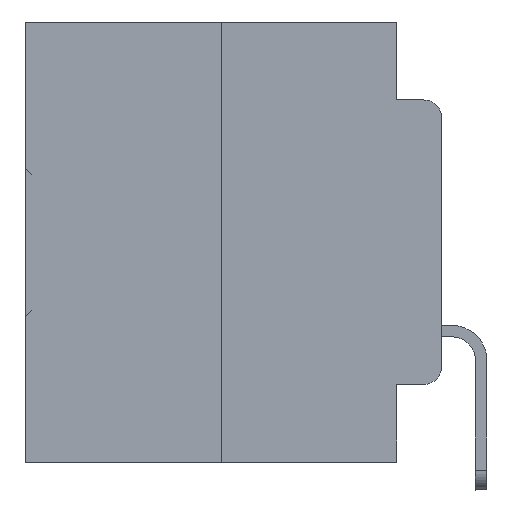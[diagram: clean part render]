
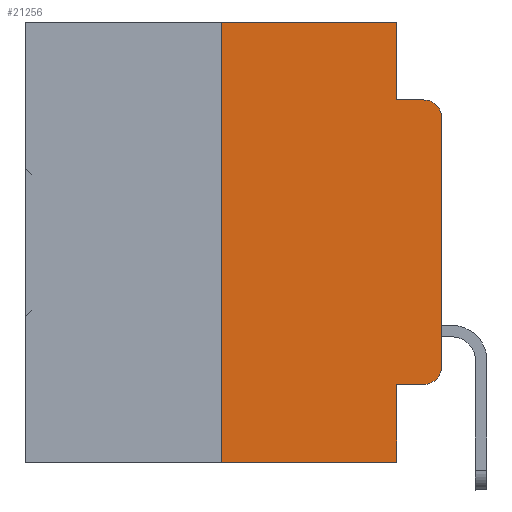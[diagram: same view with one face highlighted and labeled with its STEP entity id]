
A CAD part, left-side view. The second image highlights one B-rep face of the part: STEP entity #21256.
In plain terms, the highlighted planar face has unit normal (-1, 0, 0).
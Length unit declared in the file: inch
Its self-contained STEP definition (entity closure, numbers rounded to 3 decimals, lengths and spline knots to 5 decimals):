
#494 = CARTESIAN_POINT ( 'NONE',  ( 0., 0.02, -0.4115 ) ) ;
#692 = LINE ( 'NONE', #28196, #25234 ) ;
#1241 = CARTESIAN_POINT ( 'NONE',  ( 0., 0.25, 0. ) ) ;
#1628 = VECTOR ( 'NONE', #8132, 39.37008 ) ;
#1717 = EDGE_CURVE ( 'NONE', #23612, #13512, #17549, .T. ) ;
#2669 = EDGE_CURVE ( 'NONE', #31862, #13512, #12969, .T. ) ;
#2868 = ORIENTED_EDGE ( 'NONE', *, *, #9686, .F. ) ;
#3126 = AXIS2_PLACEMENT_3D ( 'NONE', #11331, #33373, #30530 ) ;
#3228 = FACE_OUTER_BOUND ( 'NONE', #25958, .T. ) ;
#3734 = ORIENTED_EDGE ( 'NONE', *, *, #23345, .F. ) ;
#3857 = DIRECTION ( 'NONE',  ( 0., -1., 0. ) ) ;
#3960 = VERTEX_POINT ( 'NONE', #15705 ) ;
#4089 = CIRCLE ( 'NONE', #10333, 0.02 ) ;
#4137 = DIRECTION ( 'NONE',  ( 0., 0., -1. ) ) ;
#4285 = ORIENTED_EDGE ( 'NONE', *, *, #2669, .F. ) ;
#4407 = VERTEX_POINT ( 'NONE', #11495 ) ;
#6607 = CARTESIAN_POINT ( 'NONE',  ( 0., 0.473, 0. ) ) ;
#7118 = LINE ( 'NONE', #12787, #20910 ) ;
#7383 = EDGE_CURVE ( 'NONE', #31862, #33399, #21274, .T. ) ;
#7499 = ORIENTED_EDGE ( 'NONE', *, *, #1717, .T. ) ;
#8031 = VECTOR ( 'NONE', #4137, 39.37008 ) ;
#8132 = DIRECTION ( 'NONE',  ( 0., -1., 0. ) ) ;
#8559 = PLANE ( 'NONE',  #22183 ) ;
#8773 = ORIENTED_EDGE ( 'NONE', *, *, #21470, .T. ) ;
#9200 = CARTESIAN_POINT ( 'NONE',  ( 0., 0.051, -0.4115 ) ) ;
#9288 = VECTOR ( 'NONE', #19876, 39.37008 ) ;
#9291 = CARTESIAN_POINT ( 'NONE',  ( 0., 0., 0. ) ) ;
#9639 = LINE ( 'NONE', #28285, #8031 ) ;
#9686 = EDGE_CURVE ( 'NONE', #28482, #16308, #9639, .T. ) ;
#9745 = EDGE_CURVE ( 'NONE', #4407, #3960, #33645, .T. ) ;
#9904 = CARTESIAN_POINT ( 'NONE',  ( 0., 0.473, -0.5 ) ) ;
#10333 = AXIS2_PLACEMENT_3D ( 'NONE', #20625, #31488, #17977 ) ;
#11331 = CARTESIAN_POINT ( 'NONE',  ( 0., 0.02, -0.3915 ) ) ;
#11495 = CARTESIAN_POINT ( 'NONE',  ( 0., 0., -0.3915 ) ) ;
#11615 = ORIENTED_EDGE ( 'NONE', *, *, #9745, .T. ) ;
#12239 = ORIENTED_EDGE ( 'NONE', *, *, #29049, .F. ) ;
#12787 = CARTESIAN_POINT ( 'NONE',  ( 0., 0.473, 0. ) ) ;
#12969 = LINE ( 'NONE', #23788, #27560 ) ;
#13512 = VERTEX_POINT ( 'NONE', #15761 ) ;
#13825 = VECTOR ( 'NONE', #25871, 39.37008 ) ;
#15108 = EDGE_CURVE ( 'NONE', #33399, #4407, #23554, .T. ) ;
#15705 = CARTESIAN_POINT ( 'NONE',  ( 0., 0., -0.1085 ) ) ;
#15761 = CARTESIAN_POINT ( 'NONE',  ( 0., 0.051, -0.5 ) ) ;
#16308 = VERTEX_POINT ( 'NONE', #21162 ) ;
#16527 = VECTOR ( 'NONE', #20122, 39.37008 ) ;
#16529 = CARTESIAN_POINT ( 'NONE',  ( 0., 0.051, 0. ) ) ;
#16909 = DIRECTION ( 'NONE',  ( 1., 0., 0. ) ) ;
#17265 = DIRECTION ( 'NONE',  ( 0., 0., -1. ) ) ;
#17549 = LINE ( 'NONE', #9904, #13825 ) ;
#17977 = DIRECTION ( 'NONE',  ( 0., 0., -1. ) ) ;
#18947 = ORIENTED_EDGE ( 'NONE', *, *, #32795, .F. ) ;
#19277 = CARTESIAN_POINT ( 'NONE',  ( 0., 0.25, -0.5 ) ) ;
#19876 = DIRECTION ( 'NONE',  ( 0., 0., 1. ) ) ;
#19930 = ORIENTED_EDGE ( 'NONE', *, *, #15108, .T. ) ;
#20122 = DIRECTION ( 'NONE',  ( 0., 0., 1. ) ) ;
#20289 = VERTEX_POINT ( 'NONE', #29626 ) ;
#20625 = CARTESIAN_POINT ( 'NONE',  ( 0., 0.02, -0.1085 ) ) ;
#20910 = VECTOR ( 'NONE', #35006, 39.37008 ) ;
#21162 = CARTESIAN_POINT ( 'NONE',  ( 0., 0.051, -0.0885 ) ) ;
#21256 = ADVANCED_FACE ( 'NONE', ( #3228 ), #8559, .F. ) ;
#21274 = LINE ( 'NONE', #24107, #1628 ) ;
#21470 = EDGE_CURVE ( 'NONE', #3960, #32176, #4089, .T. ) ;
#22183 = AXIS2_PLACEMENT_3D ( 'NONE', #6607, #16909, #17265 ) ;
#23345 = EDGE_CURVE ( 'NONE', #23612, #20289, #25532, .T. ) ;
#23554 = CIRCLE ( 'NONE', #3126, 0.02 ) ;
#23612 = VERTEX_POINT ( 'NONE', #19277 ) ;
#23788 = CARTESIAN_POINT ( 'NONE',  ( 0., 0.051, 0. ) ) ;
#24107 = CARTESIAN_POINT ( 'NONE',  ( 0., 0.051, -0.4115 ) ) ;
#25234 = VECTOR ( 'NONE', #3857, 39.37008 ) ;
#25532 = LINE ( 'NONE', #1241, #9288 ) ;
#25871 = DIRECTION ( 'NONE',  ( 0., -1., 0. ) ) ;
#25958 = EDGE_LOOP ( 'NONE', ( #11615, #8773, #12239, #2868, #18947, #3734, #7499, #4285, #29013, #19930 ) ) ;
#27404 = CARTESIAN_POINT ( 'NONE',  ( 0., 0.02, -0.0885 ) ) ;
#27560 = VECTOR ( 'NONE', #34655, 39.37008 ) ;
#28196 = CARTESIAN_POINT ( 'NONE',  ( 0., 0.051, -0.0885 ) ) ;
#28285 = CARTESIAN_POINT ( 'NONE',  ( 0., 0.051, 0. ) ) ;
#28482 = VERTEX_POINT ( 'NONE', #16529 ) ;
#29013 = ORIENTED_EDGE ( 'NONE', *, *, #7383, .T. ) ;
#29049 = EDGE_CURVE ( 'NONE', #16308, #32176, #692, .T. ) ;
#29626 = CARTESIAN_POINT ( 'NONE',  ( 0., 0.25, 0. ) ) ;
#30530 = DIRECTION ( 'NONE',  ( 0., 0., -1. ) ) ;
#31488 = DIRECTION ( 'NONE',  ( -1., 0., 0. ) ) ;
#31862 = VERTEX_POINT ( 'NONE', #9200 ) ;
#32176 = VERTEX_POINT ( 'NONE', #27404 ) ;
#32795 = EDGE_CURVE ( 'NONE', #20289, #28482, #7118, .T. ) ;
#33373 = DIRECTION ( 'NONE',  ( -1., 0., 0. ) ) ;
#33399 = VERTEX_POINT ( 'NONE', #494 ) ;
#33645 = LINE ( 'NONE', #9291, #16527 ) ;
#34655 = DIRECTION ( 'NONE',  ( 0., 0., -1. ) ) ;
#35006 = DIRECTION ( 'NONE',  ( 0., -1., 0. ) ) ;
